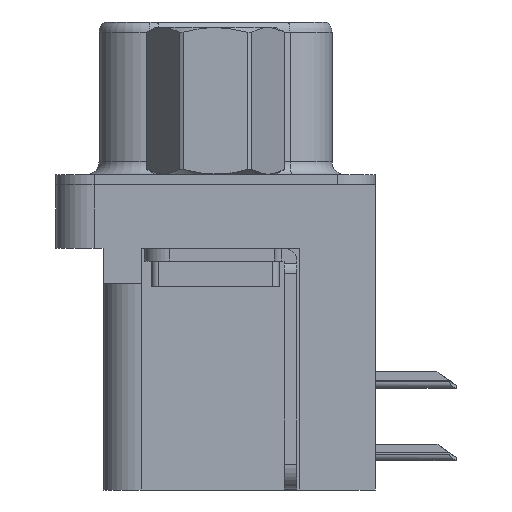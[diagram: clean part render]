
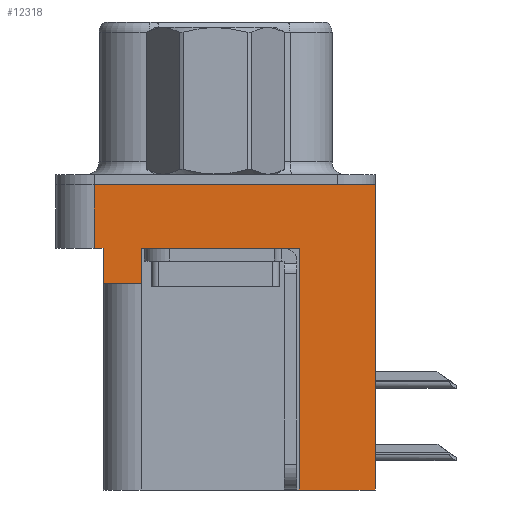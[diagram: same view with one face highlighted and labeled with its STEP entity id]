
A CAD part, left-side view. The second image highlights one B-rep face of the part: STEP entity #12318.
In plain terms, the highlighted planar face has unit normal (-1, 0, 0).
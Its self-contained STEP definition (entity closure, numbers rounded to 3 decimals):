
#86 = VERTEX_POINT ( 'NONE', #3360 ) ;
#255 = EDGE_CURVE ( 'NONE', #86, #25626, #6755, .T. ) ;
#360 = VECTOR ( 'NONE', #17446, 1000. ) ;
#882 = EDGE_CURVE ( 'NONE', #86, #21433, #1071, .T. ) ;
#892 = LINE ( 'NONE', #5357, #1297 ) ;
#950 = EDGE_CURVE ( 'NONE', #19347, #29939, #2187, .T. ) ;
#1071 = LINE ( 'NONE', #27081, #25128 ) ;
#1297 = VECTOR ( 'NONE', #15282, 1000. ) ;
#1409 = AXIS2_PLACEMENT_3D ( 'NONE', #16212, #8837, #16318 ) ;
#1875 = ORIENTED_EDGE ( 'NONE', *, *, #8316, .F. ) ;
#2187 = LINE ( 'NONE', #26848, #19078 ) ;
#2378 = VERTEX_POINT ( 'NONE', #30625 ) ;
#3208 = ORIENTED_EDGE ( 'NONE', *, *, #255, .F. ) ;
#3360 = CARTESIAN_POINT ( 'NONE',  ( -2.91, -6.275, -12. ) ) ;
#3709 = EDGE_CURVE ( 'NONE', #21278, #27541, #7213, .T. ) ;
#3787 = LINE ( 'NONE', #29679, #360 ) ;
#4186 = VECTOR ( 'NONE', #16948, 1000. ) ;
#4808 = VERTEX_POINT ( 'NONE', #5669 ) ;
#5133 = DIRECTION ( 'NONE',  ( 0., 1., 0. ) ) ;
#5357 = CARTESIAN_POINT ( 'NONE',  ( -2.91, -6.275, -2.5 ) ) ;
#5431 = CARTESIAN_POINT ( 'NONE',  ( -2.91, 4.775, -2.5 ) ) ;
#5669 = CARTESIAN_POINT ( 'NONE',  ( -2.91, 2.895, -3.9 ) ) ;
#6363 = CARTESIAN_POINT ( 'NONE',  ( -2.91, 4.425, -3.9 ) ) ;
#6755 = LINE ( 'NONE', #14740, #11423 ) ;
#7213 = LINE ( 'NONE', #31009, #12888 ) ;
#7412 = VECTOR ( 'NONE', #30195, 1000. ) ;
#7533 = FACE_OUTER_BOUND ( 'NONE', #25090, .T. ) ;
#8205 = LINE ( 'NONE', #14447, #11319 ) ;
#8316 = EDGE_CURVE ( 'NONE', #29939, #21433, #21282, .T. ) ;
#8837 = DIRECTION ( 'NONE',  ( -1., 0., 0. ) ) ;
#9201 = ORIENTED_EDGE ( 'NONE', *, *, #882, .T. ) ;
#9650 = VECTOR ( 'NONE', #18107, 1000. ) ;
#11319 = VECTOR ( 'NONE', #31404, 1000. ) ;
#11423 = VECTOR ( 'NONE', #5133, 1000. ) ;
#11525 = LINE ( 'NONE', #26788, #4186 ) ;
#12164 = DIRECTION ( 'NONE',  ( 0., 0., 1. ) ) ;
#12233 = DIRECTION ( 'NONE',  ( 0., 0., 1. ) ) ;
#12318 = ADVANCED_FACE ( 'NONE', ( #7533 ), #26056, .T. ) ;
#12671 = CARTESIAN_POINT ( 'NONE',  ( -2.91, -3.295, -2.5 ) ) ;
#12888 = VECTOR ( 'NONE', #19083, 1000. ) ;
#14447 = CARTESIAN_POINT ( 'NONE',  ( -2.91, 4.425, -3.9 ) ) ;
#14740 = CARTESIAN_POINT ( 'NONE',  ( -2.91, -3.295, -12. ) ) ;
#15282 = DIRECTION ( 'NONE',  ( 0., -1., 0. ) ) ;
#15502 = ORIENTED_EDGE ( 'NONE', *, *, #28902, .F. ) ;
#15635 = ORIENTED_EDGE ( 'NONE', *, *, #3709, .F. ) ;
#15722 = CARTESIAN_POINT ( 'NONE',  ( -2.91, -6.275, -2.5 ) ) ;
#16212 = CARTESIAN_POINT ( 'NONE',  ( -2.91, -6.275, -2.5 ) ) ;
#16318 = DIRECTION ( 'NONE',  ( 0., 0., 1. ) ) ;
#16866 = ORIENTED_EDGE ( 'NONE', *, *, #26452, .F. ) ;
#16948 = DIRECTION ( 'NONE',  ( 0., 0., 1. ) ) ;
#17446 = DIRECTION ( 'NONE',  ( 0., 0., 1. ) ) ;
#18107 = DIRECTION ( 'NONE',  ( 0., -1., 0. ) ) ;
#18233 = ORIENTED_EDGE ( 'NONE', *, *, #22888, .T. ) ;
#19078 = VECTOR ( 'NONE', #12233, 1000. ) ;
#19083 = DIRECTION ( 'NONE',  ( 0., 0., 1. ) ) ;
#19088 = CARTESIAN_POINT ( 'NONE',  ( -2.91, 4.775, 0. ) ) ;
#19347 = VERTEX_POINT ( 'NONE', #5431 ) ;
#20326 = CARTESIAN_POINT ( 'NONE',  ( -2.91, -3.295, -12. ) ) ;
#21278 = VERTEX_POINT ( 'NONE', #6363 ) ;
#21282 = LINE ( 'NONE', #27772, #7412 ) ;
#21433 = VERTEX_POINT ( 'NONE', #28239 ) ;
#21659 = EDGE_CURVE ( 'NONE', #4808, #2378, #11525, .T. ) ;
#22198 = ORIENTED_EDGE ( 'NONE', *, *, #22975, .T. ) ;
#22888 = EDGE_CURVE ( 'NONE', #19347, #27541, #892, .T. ) ;
#22975 = EDGE_CURVE ( 'NONE', #2378, #30807, #23098, .T. ) ;
#23098 = LINE ( 'NONE', #15722, #9650 ) ;
#25090 = EDGE_LOOP ( 'NONE', ( #1875, #30798, #18233, #15635, #16866, #25875, #22198, #15502, #3208, #9201 ) ) ;
#25128 = VECTOR ( 'NONE', #12164, 1000. ) ;
#25626 = VERTEX_POINT ( 'NONE', #20326 ) ;
#25875 = ORIENTED_EDGE ( 'NONE', *, *, #21659, .T. ) ;
#26056 = PLANE ( 'NONE',  #1409 ) ;
#26452 = EDGE_CURVE ( 'NONE', #4808, #21278, #8205, .T. ) ;
#26788 = CARTESIAN_POINT ( 'NONE',  ( -2.91, 2.895, -3.9 ) ) ;
#26848 = CARTESIAN_POINT ( 'NONE',  ( -2.91, 4.775, -2.5 ) ) ;
#26866 = CARTESIAN_POINT ( 'NONE',  ( -2.91, 4.425, -2.5 ) ) ;
#27081 = CARTESIAN_POINT ( 'NONE',  ( -2.91, -6.275, -2.5 ) ) ;
#27541 = VERTEX_POINT ( 'NONE', #26866 ) ;
#27772 = CARTESIAN_POINT ( 'NONE',  ( -2.91, -6.275, 0. ) ) ;
#28239 = CARTESIAN_POINT ( 'NONE',  ( -2.91, -6.275, 0. ) ) ;
#28902 = EDGE_CURVE ( 'NONE', #25626, #30807, #3787, .T. ) ;
#29679 = CARTESIAN_POINT ( 'NONE',  ( -2.91, -3.295, -12. ) ) ;
#29939 = VERTEX_POINT ( 'NONE', #19088 ) ;
#30195 = DIRECTION ( 'NONE',  ( 0., -1., 0. ) ) ;
#30625 = CARTESIAN_POINT ( 'NONE',  ( -2.91, 2.895, -2.5 ) ) ;
#30798 = ORIENTED_EDGE ( 'NONE', *, *, #950, .F. ) ;
#30807 = VERTEX_POINT ( 'NONE', #12671 ) ;
#31009 = CARTESIAN_POINT ( 'NONE',  ( -2.91, 4.425, -3.9 ) ) ;
#31404 = DIRECTION ( 'NONE',  ( 0., 1., 0. ) ) ;
